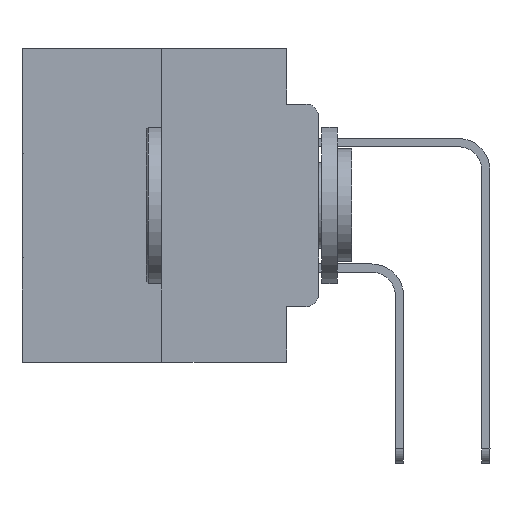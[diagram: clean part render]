
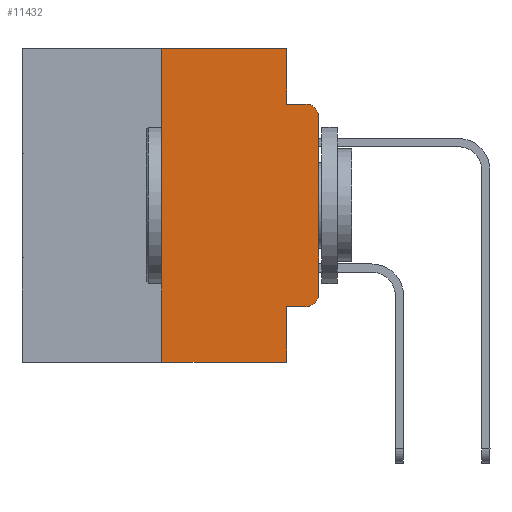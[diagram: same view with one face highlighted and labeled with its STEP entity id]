
A CAD part, left-side view. The second image highlights one B-rep face of the part: STEP entity #11432.
In plain terms, the highlighted planar face has unit normal (-1, 0, 0).
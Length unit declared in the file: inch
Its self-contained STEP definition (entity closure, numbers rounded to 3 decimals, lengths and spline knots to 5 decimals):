
#434 = ORIENTED_EDGE ( 'NONE', *, *, #8232, .F. ) ;
#747 = EDGE_CURVE ( 'NONE', #10084, #27342, #19169, .T. ) ;
#992 = CARTESIAN_POINT ( 'NONE',  ( 0., 0.051, -0.0885 ) ) ;
#1720 = VERTEX_POINT ( 'NONE', #1750 ) ;
#1750 = CARTESIAN_POINT ( 'NONE',  ( 0., 0.02, -0.0885 ) ) ;
#1778 = EDGE_LOOP ( 'NONE', ( #30190, #27181, #9894, #16370, #26262, #8194, #27365, #434, #5266, #20887 ) ) ;
#1796 = LINE ( 'NONE', #3892, #6496 ) ;
#2017 = VERTEX_POINT ( 'NONE', #13019 ) ;
#2843 = EDGE_CURVE ( 'NONE', #20171, #9239, #12788, .T. ) ;
#3406 = DIRECTION ( 'NONE',  ( 0., 0., 1. ) ) ;
#3553 = DIRECTION ( 'NONE',  ( 0., 0., -1. ) ) ;
#3580 = DIRECTION ( 'NONE',  ( 0., -1., 0. ) ) ;
#3616 = DIRECTION ( 'NONE',  ( 0., 0., -1. ) ) ;
#3892 = CARTESIAN_POINT ( 'NONE',  ( 0., 0.051, -0.4115 ) ) ;
#4713 = CARTESIAN_POINT ( 'NONE',  ( 0., 0.051, 0. ) ) ;
#5266 = ORIENTED_EDGE ( 'NONE', *, *, #17740, .T. ) ;
#5639 = FACE_OUTER_BOUND ( 'NONE', #1778, .T. ) ;
#5912 = EDGE_CURVE ( 'NONE', #2017, #10084, #13522, .T. ) ;
#6496 = VECTOR ( 'NONE', #20905, 39.37008 ) ;
#6687 = CARTESIAN_POINT ( 'NONE',  ( 0., 0.473, 0. ) ) ;
#7115 = CARTESIAN_POINT ( 'NONE',  ( 0., 0.051, 0. ) ) ;
#7391 = DIRECTION ( 'NONE',  ( 0., 0., -1. ) ) ;
#7660 = DIRECTION ( 'NONE',  ( 0., 0., 1. ) ) ;
#7689 = CARTESIAN_POINT ( 'NONE',  ( 0., 0., -0.1085 ) ) ;
#8194 = ORIENTED_EDGE ( 'NONE', *, *, #12817, .F. ) ;
#8232 = EDGE_CURVE ( 'NONE', #26757, #9239, #9498, .T. ) ;
#8259 = CARTESIAN_POINT ( 'NONE',  ( 0., 0., -0.3915 ) ) ;
#8347 = LINE ( 'NONE', #992, #16282 ) ;
#9203 = VERTEX_POINT ( 'NONE', #25964 ) ;
#9239 = VERTEX_POINT ( 'NONE', #28820 ) ;
#9498 = LINE ( 'NONE', #7115, #24363 ) ;
#9770 = DIRECTION ( 'NONE',  ( -1., 0., 0. ) ) ;
#9894 = ORIENTED_EDGE ( 'NONE', *, *, #23104, .F. ) ;
#10084 = VERTEX_POINT ( 'NONE', #21145 ) ;
#11119 = VECTOR ( 'NONE', #14386, 39.37008 ) ;
#11249 = AXIS2_PLACEMENT_3D ( 'NONE', #6687, #26088, #3553 ) ;
#11432 = ADVANCED_FACE ( 'NONE', ( #5639 ), #18013, .F. ) ;
#11661 = AXIS2_PLACEMENT_3D ( 'NONE', #26781, #9770, #7391 ) ;
#11735 = VERTEX_POINT ( 'NONE', #8259 ) ;
#12788 = LINE ( 'NONE', #17882, #13635 ) ;
#12817 = EDGE_CURVE ( 'NONE', #20171, #2017, #30117, .T. ) ;
#13019 = CARTESIAN_POINT ( 'NONE',  ( 0., 0.25, 0. ) ) ;
#13388 = CARTESIAN_POINT ( 'NONE',  ( 0., 0.25, 0. ) ) ;
#13522 = LINE ( 'NONE', #20552, #19153 ) ;
#13635 = VECTOR ( 'NONE', #3580, 39.37008 ) ;
#14164 = VECTOR ( 'NONE', #7660, 39.37008 ) ;
#14232 = DIRECTION ( 'NONE',  ( 0., 0., -1. ) ) ;
#14386 = DIRECTION ( 'NONE',  ( 0., 0., -1. ) ) ;
#14663 = CARTESIAN_POINT ( 'NONE',  ( 0., 0.25, -0.5 ) ) ;
#15830 = EDGE_CURVE ( 'NONE', #9203, #11735, #17020, .T. ) ;
#16282 = VECTOR ( 'NONE', #20098, 39.37008 ) ;
#16370 = ORIENTED_EDGE ( 'NONE', *, *, #747, .F. ) ;
#16611 = VERTEX_POINT ( 'NONE', #7689 ) ;
#17020 = CIRCLE ( 'NONE', #28720, 0.02 ) ;
#17740 = EDGE_CURVE ( 'NONE', #26757, #9203, #1796, .T. ) ;
#17882 = CARTESIAN_POINT ( 'NONE',  ( 0., 0.473, -0.5 ) ) ;
#18013 = PLANE ( 'NONE',  #11249 ) ;
#18148 = DIRECTION ( 'NONE',  ( 0., -1., 0. ) ) ;
#19153 = VECTOR ( 'NONE', #18148, 39.37008 ) ;
#19169 = LINE ( 'NONE', #4713, #11119 ) ;
#19724 = CARTESIAN_POINT ( 'NONE',  ( 0., 0., 0. ) ) ;
#20098 = DIRECTION ( 'NONE',  ( 0., -1., 0. ) ) ;
#20149 = CARTESIAN_POINT ( 'NONE',  ( 0., 0.02, -0.3915 ) ) ;
#20171 = VERTEX_POINT ( 'NONE', #14663 ) ;
#20552 = CARTESIAN_POINT ( 'NONE',  ( 0., 0.473, 0. ) ) ;
#20887 = ORIENTED_EDGE ( 'NONE', *, *, #15830, .T. ) ;
#20905 = DIRECTION ( 'NONE',  ( 0., -1., 0. ) ) ;
#21145 = CARTESIAN_POINT ( 'NONE',  ( 0., 0.051, 0. ) ) ;
#22550 = DIRECTION ( 'NONE',  ( -1., 0., 0. ) ) ;
#23104 = EDGE_CURVE ( 'NONE', #27342, #1720, #8347, .T. ) ;
#23461 = CARTESIAN_POINT ( 'NONE',  ( 0., 0.051, -0.0885 ) ) ;
#24363 = VECTOR ( 'NONE', #14232, 39.37008 ) ;
#24518 = VECTOR ( 'NONE', #3406, 39.37008 ) ;
#25364 = CIRCLE ( 'NONE', #11661, 0.02 ) ;
#25964 = CARTESIAN_POINT ( 'NONE',  ( 0., 0.02, -0.4115 ) ) ;
#26088 = DIRECTION ( 'NONE',  ( 1., 0., 0. ) ) ;
#26262 = ORIENTED_EDGE ( 'NONE', *, *, #5912, .F. ) ;
#26757 = VERTEX_POINT ( 'NONE', #26991 ) ;
#26781 = CARTESIAN_POINT ( 'NONE',  ( 0., 0.02, -0.1085 ) ) ;
#26893 = LINE ( 'NONE', #19724, #14164 ) ;
#26991 = CARTESIAN_POINT ( 'NONE',  ( 0., 0.051, -0.4115 ) ) ;
#27181 = ORIENTED_EDGE ( 'NONE', *, *, #27449, .T. ) ;
#27342 = VERTEX_POINT ( 'NONE', #23461 ) ;
#27365 = ORIENTED_EDGE ( 'NONE', *, *, #2843, .T. ) ;
#27449 = EDGE_CURVE ( 'NONE', #16611, #1720, #25364, .T. ) ;
#27941 = EDGE_CURVE ( 'NONE', #11735, #16611, #26893, .T. ) ;
#28720 = AXIS2_PLACEMENT_3D ( 'NONE', #20149, #22550, #3616 ) ;
#28820 = CARTESIAN_POINT ( 'NONE',  ( 0., 0.051, -0.5 ) ) ;
#30117 = LINE ( 'NONE', #13388, #24518 ) ;
#30190 = ORIENTED_EDGE ( 'NONE', *, *, #27941, .T. ) ;
